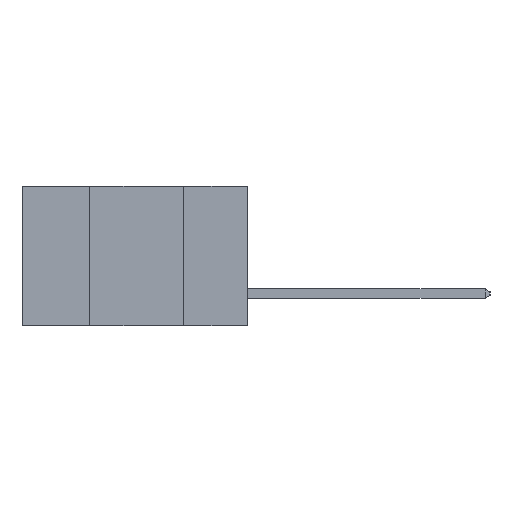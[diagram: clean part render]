
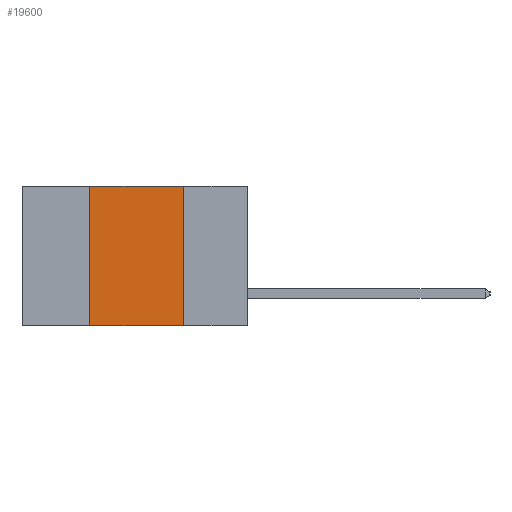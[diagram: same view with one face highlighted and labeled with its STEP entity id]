
A CAD part, left-side view. The second image highlights one B-rep face of the part: STEP entity #19600.
In plain terms, the highlighted planar face has unit normal (-1, 0, 0).
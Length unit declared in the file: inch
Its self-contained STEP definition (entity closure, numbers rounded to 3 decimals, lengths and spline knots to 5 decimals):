
#2040 = CARTESIAN_POINT ( 'NONE',  ( 0., 0.42, 0. ) ) ;
#2113 = ORIENTED_EDGE ( 'NONE', *, *, #30847, .F. ) ;
#2138 = LINE ( 'NONE', #2040, #7934 ) ;
#3534 = AXIS2_PLACEMENT_3D ( 'NONE', #23735, #9191, #26139 ) ;
#4111 = VECTOR ( 'NONE', #6299, 39.37008 ) ;
#6299 = DIRECTION ( 'NONE',  ( 0., 0., -1. ) ) ;
#6470 = VERTEX_POINT ( 'NONE', #30561 ) ;
#7934 = VECTOR ( 'NONE', #16663, 39.37008 ) ;
#7955 = EDGE_LOOP ( 'NONE', ( #29220, #16042, #2113, #25284 ) ) ;
#8402 = LINE ( 'NONE', #22483, #21304 ) ;
#8672 = CARTESIAN_POINT ( 'NONE',  ( 0., 0.17, 0. ) ) ;
#9085 = PLANE ( 'NONE',  #3534 ) ;
#9191 = DIRECTION ( 'NONE',  ( 1., 0., 0. ) ) ;
#10075 = VECTOR ( 'NONE', #30862, 39.37008 ) ;
#10328 = DIRECTION ( 'NONE',  ( 0., -1., 0. ) ) ;
#10697 = VERTEX_POINT ( 'NONE', #24018 ) ;
#10818 = LINE ( 'NONE', #28507, #10075 ) ;
#14668 = FACE_OUTER_BOUND ( 'NONE', #7955, .T. ) ;
#15738 = EDGE_CURVE ( 'NONE', #25666, #19817, #23576, .T. ) ;
#16042 = ORIENTED_EDGE ( 'NONE', *, *, #23475, .F. ) ;
#16663 = DIRECTION ( 'NONE',  ( 0., 0., 1. ) ) ;
#17263 = CARTESIAN_POINT ( 'NONE',  ( 0., 0.17, -0.37 ) ) ;
#19600 = ADVANCED_FACE ( 'NONE', ( #14668 ), #9085, .F. ) ;
#19817 = VERTEX_POINT ( 'NONE', #17263 ) ;
#21304 = VECTOR ( 'NONE', #10328, 39.37008 ) ;
#22214 = CARTESIAN_POINT ( 'NONE',  ( 0., 0.17, 0. ) ) ;
#22483 = CARTESIAN_POINT ( 'NONE',  ( 0., 0.6, 0. ) ) ;
#23475 = EDGE_CURVE ( 'NONE', #10697, #25666, #8402, .T. ) ;
#23576 = LINE ( 'NONE', #8672, #4111 ) ;
#23735 = CARTESIAN_POINT ( 'NONE',  ( 0., 0.6, 0. ) ) ;
#24018 = CARTESIAN_POINT ( 'NONE',  ( 0., 0.42, 0. ) ) ;
#25284 = ORIENTED_EDGE ( 'NONE', *, *, #26058, .T. ) ;
#25666 = VERTEX_POINT ( 'NONE', #22214 ) ;
#26058 = EDGE_CURVE ( 'NONE', #6470, #19817, #10818, .T. ) ;
#26139 = DIRECTION ( 'NONE',  ( 0., 0., -1. ) ) ;
#28507 = CARTESIAN_POINT ( 'NONE',  ( 0., 0.6, -0.37 ) ) ;
#29220 = ORIENTED_EDGE ( 'NONE', *, *, #15738, .F. ) ;
#30561 = CARTESIAN_POINT ( 'NONE',  ( 0., 0.42, -0.37 ) ) ;
#30847 = EDGE_CURVE ( 'NONE', #6470, #10697, #2138, .T. ) ;
#30862 = DIRECTION ( 'NONE',  ( 0., -1., 0. ) ) ;
